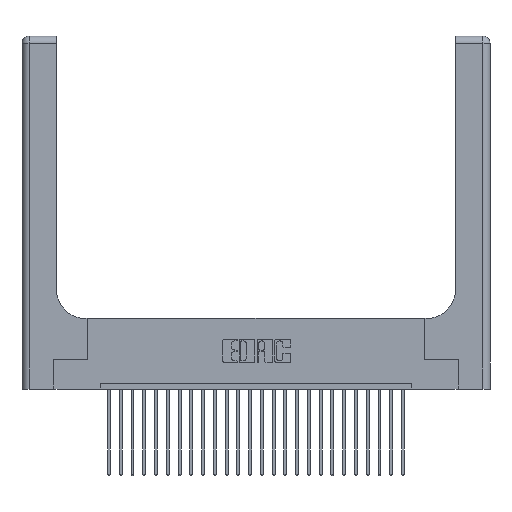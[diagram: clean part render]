
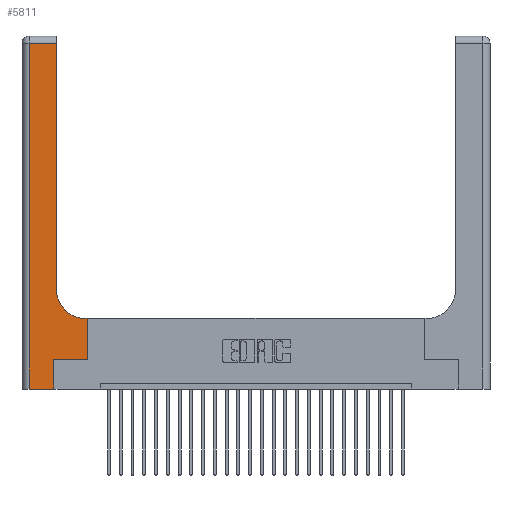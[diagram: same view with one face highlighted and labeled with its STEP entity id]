
A CAD part, top view. The second image highlights one B-rep face of the part: STEP entity #5811.
In plain terms, the highlighted planar face has unit normal (0, 0, 1).
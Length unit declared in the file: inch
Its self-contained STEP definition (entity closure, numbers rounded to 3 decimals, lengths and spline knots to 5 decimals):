
#377 = VERTEX_POINT ( 'NONE', #11913 ) ;
#541 = ORIENTED_EDGE ( 'NONE', *, *, #16402, .T. ) ;
#967 = CARTESIAN_POINT ( 'NONE',  ( 0.5415, 0.6, 0.37 ) ) ;
#1212 = PLANE ( 'NONE',  #1783 ) ;
#1250 = ORIENTED_EDGE ( 'NONE', *, *, #24379, .T. ) ;
#1395 = VECTOR ( 'NONE', #18113, 39.37008 ) ;
#1783 = AXIS2_PLACEMENT_3D ( 'NONE', #15722, #25935, #13655 ) ;
#2294 = LINE ( 'NONE', #4741, #11492 ) ;
#2390 = CARTESIAN_POINT ( 'NONE',  ( 0.269, 0., 0.37 ) ) ;
#2800 = CARTESIAN_POINT ( 'NONE',  ( 0.269, 0.25, 0.37 ) ) ;
#2907 = DIRECTION ( 'NONE',  ( -1., 0., 0. ) ) ;
#3129 = EDGE_CURVE ( 'NONE', #17759, #19011, #8055, .T. ) ;
#4103 = EDGE_CURVE ( 'NONE', #13879, #17801, #10664, .T. ) ;
#4146 = ORIENTED_EDGE ( 'NONE', *, *, #4103, .T. ) ;
#4335 = CARTESIAN_POINT ( 'NONE',  ( 0.5585, 0.25, 0.37 ) ) ;
#4741 = CARTESIAN_POINT ( 'NONE',  ( 0.2915, 0.6, 0.37 ) ) ;
#5811 = ADVANCED_FACE ( 'NONE', ( #15487 ), #1212, .F. ) ;
#5975 = AXIS2_PLACEMENT_3D ( 'NONE', #12106, #16259, #10416 ) ;
#6222 = DIRECTION ( 'NONE',  ( 0., 1., 0. ) ) ;
#6541 = EDGE_CURVE ( 'NONE', #19011, #377, #18955, .T. ) ;
#6625 = VECTOR ( 'NONE', #25699, 39.37008 ) ;
#7092 = VECTOR ( 'NONE', #12973, 39.37008 ) ;
#7897 = DIRECTION ( 'NONE',  ( 0., -1., 0. ) ) ;
#8055 = LINE ( 'NONE', #11315, #15255 ) ;
#8944 = ORIENTED_EDGE ( 'NONE', *, *, #16864, .T. ) ;
#9208 = CARTESIAN_POINT ( 'NONE',  ( 0., 2.94, 0.37 ) ) ;
#10081 = LINE ( 'NONE', #20773, #25676 ) ;
#10416 = DIRECTION ( 'NONE',  ( 1., 0., 0. ) ) ;
#10664 = LINE ( 'NONE', #14958, #7092 ) ;
#10723 = DIRECTION ( 'NONE',  ( 0., 1., 0. ) ) ;
#11315 = CARTESIAN_POINT ( 'NONE',  ( 0.2915, 3., 0.37 ) ) ;
#11350 = ORIENTED_EDGE ( 'NONE', *, *, #12889, .T. ) ;
#11351 = CARTESIAN_POINT ( 'NONE',  ( 0.5585, 0.6, 0.37 ) ) ;
#11492 = VECTOR ( 'NONE', #2907, 39.37008 ) ;
#11506 = CARTESIAN_POINT ( 'NONE',  ( 0.06, 0., 0.37 ) ) ;
#11838 = EDGE_CURVE ( 'NONE', #25408, #25933, #2294, .T. ) ;
#11913 = CARTESIAN_POINT ( 'NONE',  ( 0.06, 2.94, 0.37 ) ) ;
#12106 = CARTESIAN_POINT ( 'NONE',  ( 0.5415, 0.85, 0.37 ) ) ;
#12109 = CARTESIAN_POINT ( 'NONE',  ( 0.2915, 0.85, 0.37 ) ) ;
#12144 = ORIENTED_EDGE ( 'NONE', *, *, #6541, .T. ) ;
#12526 = ORIENTED_EDGE ( 'NONE', *, *, #22884, .T. ) ;
#12889 = EDGE_CURVE ( 'NONE', #25933, #17759, #23734, .T. ) ;
#12973 = DIRECTION ( 'NONE',  ( 1., 0., 0. ) ) ;
#13655 = DIRECTION ( 'NONE',  ( -1., 0., 0. ) ) ;
#13796 = VERTEX_POINT ( 'NONE', #18720 ) ;
#13879 = VERTEX_POINT ( 'NONE', #11506 ) ;
#14958 = CARTESIAN_POINT ( 'NONE',  ( 0., 0., 0.37 ) ) ;
#15255 = VECTOR ( 'NONE', #19654, 39.37008 ) ;
#15487 = FACE_OUTER_BOUND ( 'NONE', #22343, .T. ) ;
#15722 = CARTESIAN_POINT ( 'NONE',  ( 0., 3., 0.37 ) ) ;
#16259 = DIRECTION ( 'NONE',  ( 0., 0., -1. ) ) ;
#16396 = VERTEX_POINT ( 'NONE', #20868 ) ;
#16402 = EDGE_CURVE ( 'NONE', #13796, #16396, #19015, .T. ) ;
#16864 = EDGE_CURVE ( 'NONE', #377, #13879, #23585, .T. ) ;
#17450 = VECTOR ( 'NONE', #10723, 39.37008 ) ;
#17738 = ORIENTED_EDGE ( 'NONE', *, *, #11838, .T. ) ;
#17759 = VERTEX_POINT ( 'NONE', #12109 ) ;
#17801 = VERTEX_POINT ( 'NONE', #2390 ) ;
#18113 = DIRECTION ( 'NONE',  ( -1., 0., 0. ) ) ;
#18720 = CARTESIAN_POINT ( 'NONE',  ( 0.269, 0.25, 0.37 ) ) ;
#18736 = LINE ( 'NONE', #4335, #17450 ) ;
#18955 = LINE ( 'NONE', #9208, #1395 ) ;
#19011 = VERTEX_POINT ( 'NONE', #23718 ) ;
#19015 = LINE ( 'NONE', #2800, #6625 ) ;
#19654 = DIRECTION ( 'NONE',  ( 0., 1., 0. ) ) ;
#20615 = CARTESIAN_POINT ( 'NONE',  ( 0.06, 3., 0.37 ) ) ;
#20773 = CARTESIAN_POINT ( 'NONE',  ( 0.269, 0., 0.37 ) ) ;
#20868 = CARTESIAN_POINT ( 'NONE',  ( 0.5585, 0.25, 0.37 ) ) ;
#22343 = EDGE_LOOP ( 'NONE', ( #26226, #12144, #8944, #4146, #1250, #541, #12526, #17738, #11350 ) ) ;
#22884 = EDGE_CURVE ( 'NONE', #16396, #25408, #18736, .T. ) ;
#23585 = LINE ( 'NONE', #20615, #25181 ) ;
#23718 = CARTESIAN_POINT ( 'NONE',  ( 0.2915, 2.94, 0.37 ) ) ;
#23734 = CIRCLE ( 'NONE', #5975, 0.25 ) ;
#24379 = EDGE_CURVE ( 'NONE', #17801, #13796, #10081, .T. ) ;
#25181 = VECTOR ( 'NONE', #7897, 39.37008 ) ;
#25408 = VERTEX_POINT ( 'NONE', #11351 ) ;
#25676 = VECTOR ( 'NONE', #6222, 39.37008 ) ;
#25699 = DIRECTION ( 'NONE',  ( 1., 0., 0. ) ) ;
#25933 = VERTEX_POINT ( 'NONE', #967 ) ;
#25935 = DIRECTION ( 'NONE',  ( 0., 0., -1. ) ) ;
#26226 = ORIENTED_EDGE ( 'NONE', *, *, #3129, .T. ) ;
